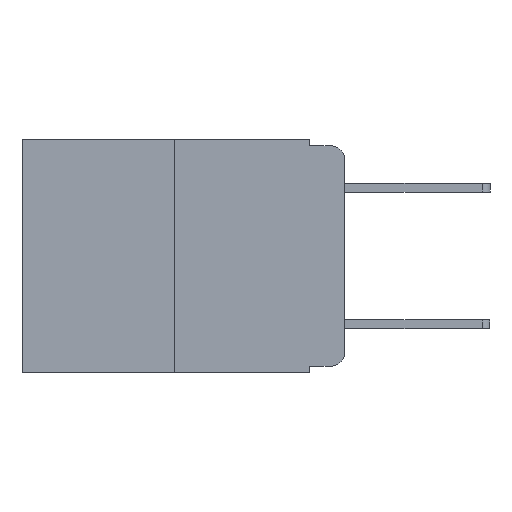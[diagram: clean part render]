
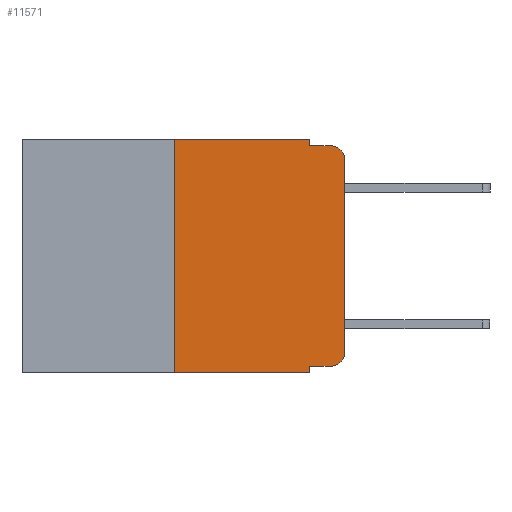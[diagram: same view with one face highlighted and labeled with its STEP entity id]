
A CAD part, left-side view. The second image highlights one B-rep face of the part: STEP entity #11571.
In plain terms, the highlighted planar face has unit normal (-1, 0, 0).
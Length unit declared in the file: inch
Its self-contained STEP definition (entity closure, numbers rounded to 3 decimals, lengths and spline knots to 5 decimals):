
#151 = CARTESIAN_POINT ( 'NONE',  ( 0., 0.051, 0. ) ) ;
#447 = VECTOR ( 'NONE', #11362, 39.37008 ) ;
#600 = VERTEX_POINT ( 'NONE', #22201 ) ;
#802 = CARTESIAN_POINT ( 'NONE',  ( 0., 0.25, -0.343 ) ) ;
#1192 = LINE ( 'NONE', #5394, #9926 ) ;
#1491 = EDGE_CURVE ( 'NONE', #600, #12707, #1192, .T. ) ;
#1668 = CARTESIAN_POINT ( 'NONE',  ( 0., 0., -0.03 ) ) ;
#2052 = CARTESIAN_POINT ( 'NONE',  ( 0., 0.051, -0.343 ) ) ;
#2308 = AXIS2_PLACEMENT_3D ( 'NONE', #19376, #8876, #21191 ) ;
#2343 = VERTEX_POINT ( 'NONE', #2052 ) ;
#2369 = CIRCLE ( 'NONE', #2308, 0.02 ) ;
#2744 = AXIS2_PLACEMENT_3D ( 'NONE', #18399, #7904, #20167 ) ;
#2777 = DIRECTION ( 'NONE',  ( 0., 0., 1. ) ) ;
#3289 = VERTEX_POINT ( 'NONE', #3342 ) ;
#3318 = VECTOR ( 'NONE', #5469, 39.37008 ) ;
#3342 = CARTESIAN_POINT ( 'NONE',  ( 0., 0.02, -0.01 ) ) ;
#3686 = DIRECTION ( 'NONE',  ( 0., 0., -1. ) ) ;
#3693 = EDGE_CURVE ( 'NONE', #21590, #6495, #6063, .T. ) ;
#3813 = LINE ( 'NONE', #13249, #18337 ) ;
#3875 = LINE ( 'NONE', #17716, #3318 ) ;
#3909 = ORIENTED_EDGE ( 'NONE', *, *, #11577, .F. ) ;
#4046 = CARTESIAN_POINT ( 'NONE',  ( 0., 0.051, 0. ) ) ;
#4121 = ORIENTED_EDGE ( 'NONE', *, *, #12390, .T. ) ;
#4358 = EDGE_LOOP ( 'NONE', ( #13450, #15815, #12815, #17341, #7987, #3909, #13673, #14652, #4121, #12171 ) ) ;
#4910 = VERTEX_POINT ( 'NONE', #20343 ) ;
#5143 = LINE ( 'NONE', #14460, #447 ) ;
#5219 = VECTOR ( 'NONE', #3686, 39.37008 ) ;
#5394 = CARTESIAN_POINT ( 'NONE',  ( 0., 0.473, 0. ) ) ;
#5469 = DIRECTION ( 'NONE',  ( 0., -1., 0. ) ) ;
#6063 = LINE ( 'NONE', #7966, #14842 ) ;
#6182 = EDGE_CURVE ( 'NONE', #4910, #2343, #5143, .T. ) ;
#6236 = DIRECTION ( 'NONE',  ( 0., 0., -1. ) ) ;
#6495 = VERTEX_POINT ( 'NONE', #1668 ) ;
#6651 = CARTESIAN_POINT ( 'NONE',  ( 0., 0.051, -0.333 ) ) ;
#7267 = CARTESIAN_POINT ( 'NONE',  ( 0., 0.02, -0.333 ) ) ;
#7904 = DIRECTION ( 'NONE',  ( -1., 0., 0. ) ) ;
#7966 = CARTESIAN_POINT ( 'NONE',  ( 0., 0., 0. ) ) ;
#7987 = ORIENTED_EDGE ( 'NONE', *, *, #1491, .F. ) ;
#8457 = VERTEX_POINT ( 'NONE', #14166 ) ;
#8876 = DIRECTION ( 'NONE',  ( -1., 0., 0. ) ) ;
#9174 = CIRCLE ( 'NONE', #2744, 0.02 ) ;
#9926 = VECTOR ( 'NONE', #20783, 39.37008 ) ;
#10653 = VERTEX_POINT ( 'NONE', #7267 ) ;
#11362 = DIRECTION ( 'NONE',  ( 0., 0., -1. ) ) ;
#11571 = ADVANCED_FACE ( 'NONE', ( #13113 ), #14902, .F. ) ;
#11577 = EDGE_CURVE ( 'NONE', #12835, #600, #3813, .T. ) ;
#11694 = AXIS2_PLACEMENT_3D ( 'NONE', #13167, #16718, #6236 ) ;
#11949 = EDGE_CURVE ( 'NONE', #12707, #8457, #19181, .T. ) ;
#12171 = ORIENTED_EDGE ( 'NONE', *, *, #18700, .T. ) ;
#12390 = EDGE_CURVE ( 'NONE', #4910, #10653, #18900, .T. ) ;
#12707 = VERTEX_POINT ( 'NONE', #4046 ) ;
#12815 = ORIENTED_EDGE ( 'NONE', *, *, #22227, .F. ) ;
#12835 = VERTEX_POINT ( 'NONE', #802 ) ;
#13113 = FACE_OUTER_BOUND ( 'NONE', #4358, .T. ) ;
#13152 = DIRECTION ( 'NONE',  ( 0., 0., 1. ) ) ;
#13167 = CARTESIAN_POINT ( 'NONE',  ( 0., 0.473, 0. ) ) ;
#13249 = CARTESIAN_POINT ( 'NONE',  ( 0., 0.25, 0. ) ) ;
#13450 = ORIENTED_EDGE ( 'NONE', *, *, #3693, .T. ) ;
#13673 = ORIENTED_EDGE ( 'NONE', *, *, #21695, .T. ) ;
#14166 = CARTESIAN_POINT ( 'NONE',  ( 0., 0.051, -0.01 ) ) ;
#14435 = DIRECTION ( 'NONE',  ( 0., -1., 0. ) ) ;
#14460 = CARTESIAN_POINT ( 'NONE',  ( 0., 0.051, 0. ) ) ;
#14652 = ORIENTED_EDGE ( 'NONE', *, *, #6182, .F. ) ;
#14842 = VECTOR ( 'NONE', #13152, 39.37008 ) ;
#14902 = PLANE ( 'NONE',  #11694 ) ;
#15815 = ORIENTED_EDGE ( 'NONE', *, *, #19081, .T. ) ;
#15897 = CARTESIAN_POINT ( 'NONE',  ( 0., 0., -0.313 ) ) ;
#16718 = DIRECTION ( 'NONE',  ( 1., 0., 0. ) ) ;
#17068 = DIRECTION ( 'NONE',  ( 0., -1., 0. ) ) ;
#17341 = ORIENTED_EDGE ( 'NONE', *, *, #11949, .F. ) ;
#17716 = CARTESIAN_POINT ( 'NONE',  ( 0., 0.051, -0.01 ) ) ;
#17800 = VECTOR ( 'NONE', #17068, 39.37008 ) ;
#17868 = VECTOR ( 'NONE', #14435, 39.37008 ) ;
#18337 = VECTOR ( 'NONE', #2777, 39.37008 ) ;
#18399 = CARTESIAN_POINT ( 'NONE',  ( 0., 0.02, -0.313 ) ) ;
#18420 = LINE ( 'NONE', #19716, #17868 ) ;
#18700 = EDGE_CURVE ( 'NONE', #10653, #21590, #9174, .T. ) ;
#18900 = LINE ( 'NONE', #6651, #17800 ) ;
#19081 = EDGE_CURVE ( 'NONE', #6495, #3289, #2369, .T. ) ;
#19181 = LINE ( 'NONE', #151, #5219 ) ;
#19376 = CARTESIAN_POINT ( 'NONE',  ( 0., 0.02, -0.03 ) ) ;
#19716 = CARTESIAN_POINT ( 'NONE',  ( 0., 0.473, -0.343 ) ) ;
#20167 = DIRECTION ( 'NONE',  ( 0., 0., -1. ) ) ;
#20343 = CARTESIAN_POINT ( 'NONE',  ( 0., 0.051, -0.333 ) ) ;
#20783 = DIRECTION ( 'NONE',  ( 0., -1., 0. ) ) ;
#21191 = DIRECTION ( 'NONE',  ( 0., 0., -1. ) ) ;
#21590 = VERTEX_POINT ( 'NONE', #15897 ) ;
#21695 = EDGE_CURVE ( 'NONE', #12835, #2343, #18420, .T. ) ;
#22201 = CARTESIAN_POINT ( 'NONE',  ( 0., 0.25, 0. ) ) ;
#22227 = EDGE_CURVE ( 'NONE', #8457, #3289, #3875, .T. ) ;
